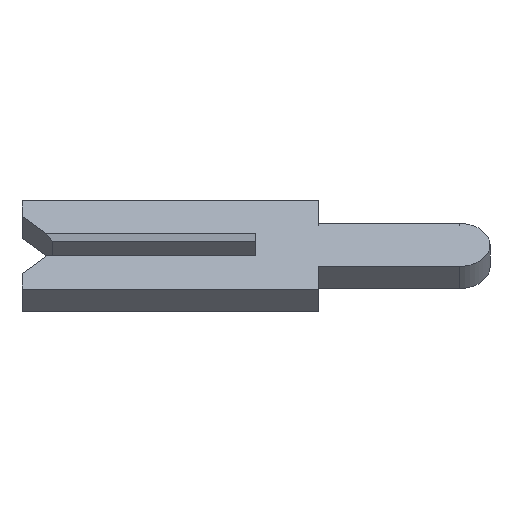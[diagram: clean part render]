
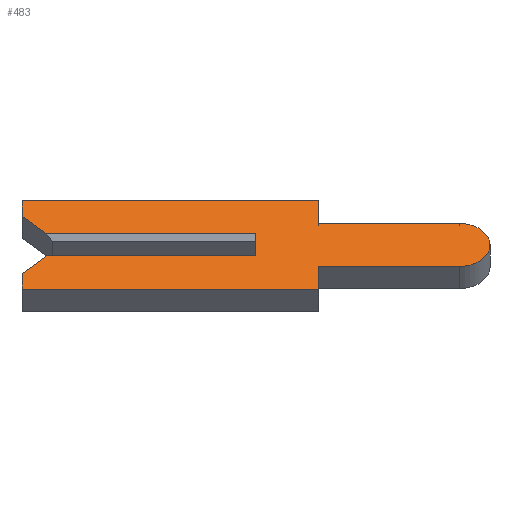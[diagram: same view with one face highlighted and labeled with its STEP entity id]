
A CAD part, left-side view. The second image highlights one B-rep face of the part: STEP entity #483.
In plain terms, the highlighted face is planar.
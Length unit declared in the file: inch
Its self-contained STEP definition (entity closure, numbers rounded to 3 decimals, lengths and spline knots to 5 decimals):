
#17 = LINE ( 'NONE', #976, #556 ) ;
#19 = DIRECTION ( 'NONE',  ( 0., 0., 1. ) ) ;
#25 = VECTOR ( 'NONE', #899, 39.37008 ) ;
#27 = CARTESIAN_POINT ( 'NONE',  ( -0.01, 0.1305, -0.0065 ) ) ;
#33 = VERTEX_POINT ( 'NONE', #515 ) ;
#41 = LINE ( 'NONE', #292, #130 ) ;
#45 = VECTOR ( 'NONE', #214, 39.37008 ) ;
#46 = EDGE_LOOP ( 'NONE', ( #150, #789, #1034, #420, #345, #579, #1049, #312, #749, #399, #894, #68, #518, #466 ) ) ;
#61 = AXIS2_PLACEMENT_3D ( 'NONE', #661, #928, #525 ) ;
#62 = EDGE_CURVE ( 'NONE', #847, #322, #457, .T. ) ;
#68 = ORIENTED_EDGE ( 'NONE', *, *, #182, .F. ) ;
#73 = CARTESIAN_POINT ( 'NONE',  ( -0.01, -0.04, 0.0195 ) ) ;
#76 = CARTESIAN_POINT ( 'NONE',  ( -0.01, -0.04, -0.0195 ) ) ;
#97 = EDGE_CURVE ( 'NONE', #671, #924, #884, .T. ) ;
#107 = CARTESIAN_POINT ( 'NONE',  ( -0.01, -0.04, 0.0195 ) ) ;
#108 = VERTEX_POINT ( 'NONE', #359 ) ;
#111 = DIRECTION ( 'NONE',  ( 0., -0.707, 0.707 ) ) ;
#122 = CARTESIAN_POINT ( 'NONE',  ( -0.01, -0.1305, 0.0195 ) ) ;
#126 = FACE_OUTER_BOUND ( 'NONE', #46, .T. ) ;
#130 = VECTOR ( 'NONE', #450, 39.37008 ) ;
#150 = ORIENTED_EDGE ( 'NONE', *, *, #632, .T. ) ;
#168 = DIRECTION ( 'NONE',  ( 0., 0., -1. ) ) ;
#177 = CARTESIAN_POINT ( 'NONE',  ( -0.01, -0.04, -0.0195 ) ) ;
#182 = EDGE_CURVE ( 'NONE', #686, #671, #241, .T. ) ;
#196 = EDGE_CURVE ( 'NONE', #33, #621, #849, .T. ) ;
#202 = VECTOR ( 'NONE', #812, 39.37008 ) ;
#214 = DIRECTION ( 'NONE',  ( 0., -1., 0. ) ) ;
#241 = LINE ( 'NONE', #433, #998 ) ;
#254 = VECTOR ( 'NONE', #352, 39.37008 ) ;
#264 = DIRECTION ( 'NONE',  ( 0., 1., 0. ) ) ;
#290 = CARTESIAN_POINT ( 'NONE',  ( -0.01, 0.15, -0.04 ) ) ;
#291 = CARTESIAN_POINT ( 'NONE',  ( -0.01, 0., 0.0065 ) ) ;
#292 = CARTESIAN_POINT ( 'NONE',  ( -0.01, 0.15, 0.026 ) ) ;
#309 = EDGE_CURVE ( 'NONE', #108, #686, #41, .T. ) ;
#312 = ORIENTED_EDGE ( 'NONE', *, *, #571, .F. ) ;
#322 = VERTEX_POINT ( 'NONE', #872 ) ;
#328 = CARTESIAN_POINT ( 'NONE',  ( -0.01, 0.134, 0.01 ) ) ;
#345 = ORIENTED_EDGE ( 'NONE', *, *, #1066, .F. ) ;
#352 = DIRECTION ( 'NONE',  ( 0., 1., 0. ) ) ;
#359 = CARTESIAN_POINT ( 'NONE',  ( -0.01, 0.15, 0.026 ) ) ;
#363 = CARTESIAN_POINT ( 'NONE',  ( -0.01, -0.1305, -0.0195 ) ) ;
#395 = PLANE ( 'NONE',  #596 ) ;
#399 = ORIENTED_EDGE ( 'NONE', *, *, #594, .F. ) ;
#420 = ORIENTED_EDGE ( 'NONE', *, *, #1006, .F. ) ;
#421 = VERTEX_POINT ( 'NONE', #122 ) ;
#430 = VECTOR ( 'NONE', #1085, 39.37008 ) ;
#433 = CARTESIAN_POINT ( 'NONE',  ( -0.01, 0.15, 0.04 ) ) ;
#434 = EDGE_CURVE ( 'NONE', #479, #108, #929, .T. ) ;
#450 = DIRECTION ( 'NONE',  ( 0., 0., 1. ) ) ;
#457 = LINE ( 'NONE', #1031, #767 ) ;
#460 = CARTESIAN_POINT ( 'NONE',  ( -0.01, -0.1305, -0.01 ) ) ;
#466 = ORIENTED_EDGE ( 'NONE', *, *, #434, .F. ) ;
#479 = VERTEX_POINT ( 'NONE', #328 ) ;
#483 = ADVANCED_FACE ( 'NONE', ( #126 ), #395, .F. ) ;
#485 = DIRECTION ( 'NONE',  ( 1., 0., 0. ) ) ;
#505 = VECTOR ( 'NONE', #111, 39.37008 ) ;
#514 = VECTOR ( 'NONE', #264, 39.37008 ) ;
#515 = CARTESIAN_POINT ( 'NONE',  ( -0.01, 0., -0.01 ) ) ;
#518 = ORIENTED_EDGE ( 'NONE', *, *, #309, .F. ) ;
#519 = VERTEX_POINT ( 'NONE', #915 ) ;
#522 = VECTOR ( 'NONE', #19, 39.37008 ) ;
#525 = DIRECTION ( 'NONE',  ( 0., 0., -1. ) ) ;
#553 = CARTESIAN_POINT ( 'NONE',  ( -0.01, 0.1305, 0.0065 ) ) ;
#556 = VECTOR ( 'NONE', #869, 39.37008 ) ;
#568 = CARTESIAN_POINT ( 'NONE',  ( -0.01, 0., 0.01 ) ) ;
#571 = EDGE_CURVE ( 'NONE', #941, #847, #645, .T. ) ;
#579 = ORIENTED_EDGE ( 'NONE', *, *, #1028, .F. ) ;
#594 = EDGE_CURVE ( 'NONE', #924, #421, #746, .T. ) ;
#595 = DIRECTION ( 'NONE',  ( 0., 0., -1. ) ) ;
#596 = AXIS2_PLACEMENT_3D ( 'NONE', #985, #485, #168 ) ;
#621 = VERTEX_POINT ( 'NONE', #568 ) ;
#632 = EDGE_CURVE ( 'NONE', #479, #621, #799, .T. ) ;
#645 = LINE ( 'NONE', #76, #514 ) ;
#647 = VECTOR ( 'NONE', #595, 39.37008 ) ;
#661 = CARTESIAN_POINT ( 'NONE',  ( -0.01, -0.1305, 0. ) ) ;
#671 = VERTEX_POINT ( 'NONE', #729 ) ;
#675 = CARTESIAN_POINT ( 'NONE',  ( -0.01, 0.134, -0.01 ) ) ;
#686 = VERTEX_POINT ( 'NONE', #922 ) ;
#729 = CARTESIAN_POINT ( 'NONE',  ( -0.01, -0.04, 0.04 ) ) ;
#746 = LINE ( 'NONE', #73, #202 ) ;
#749 = ORIENTED_EDGE ( 'NONE', *, *, #840, .F. ) ;
#756 = CARTESIAN_POINT ( 'NONE',  ( -0.01, -0.04, 0.04 ) ) ;
#762 = CARTESIAN_POINT ( 'NONE',  ( -0.01, 0.15, -0.026 ) ) ;
#767 = VECTOR ( 'NONE', #1042, 39.37008 ) ;
#778 = CIRCLE ( 'NONE', #61, 0.0195 ) ;
#789 = ORIENTED_EDGE ( 'NONE', *, *, #196, .F. ) ;
#799 = LINE ( 'NONE', #908, #430 ) ;
#812 = DIRECTION ( 'NONE',  ( 0., -1., 0. ) ) ;
#840 = EDGE_CURVE ( 'NONE', #421, #941, #778, .T. ) ;
#847 = VERTEX_POINT ( 'NONE', #177 ) ;
#849 = LINE ( 'NONE', #291, #522 ) ;
#862 = VERTEX_POINT ( 'NONE', #762 ) ;
#869 = DIRECTION ( 'NONE',  ( 0., 0., 1. ) ) ;
#872 = CARTESIAN_POINT ( 'NONE',  ( -0.01, -0.04, -0.04 ) ) ;
#884 = LINE ( 'NONE', #756, #647 ) ;
#894 = ORIENTED_EDGE ( 'NONE', *, *, #97, .F. ) ;
#899 = DIRECTION ( 'NONE',  ( 0., 0.707, 0.707 ) ) ;
#908 = CARTESIAN_POINT ( 'NONE',  ( -0.01, 0.15, 0.01 ) ) ;
#915 = CARTESIAN_POINT ( 'NONE',  ( -0.01, 0.15, -0.04 ) ) ;
#922 = CARTESIAN_POINT ( 'NONE',  ( -0.01, 0.15, 0.04 ) ) ;
#924 = VERTEX_POINT ( 'NONE', #107 ) ;
#925 = VERTEX_POINT ( 'NONE', #675 ) ;
#928 = DIRECTION ( 'NONE',  ( 1., 0., 0. ) ) ;
#929 = LINE ( 'NONE', #553, #25 ) ;
#940 = DIRECTION ( 'NONE',  ( 0., -1., 0. ) ) ;
#941 = VERTEX_POINT ( 'NONE', #363 ) ;
#967 = LINE ( 'NONE', #27, #505 ) ;
#976 = CARTESIAN_POINT ( 'NONE',  ( -0.01, 0.15, -0.026 ) ) ;
#985 = CARTESIAN_POINT ( 'NONE',  ( -0.01, -0.1305, 0. ) ) ;
#998 = VECTOR ( 'NONE', #940, 39.37008 ) ;
#1006 = EDGE_CURVE ( 'NONE', #862, #925, #967, .T. ) ;
#1015 = LINE ( 'NONE', #460, #45 ) ;
#1028 = EDGE_CURVE ( 'NONE', #322, #519, #1052, .T. ) ;
#1031 = CARTESIAN_POINT ( 'NONE',  ( -0.01, -0.04, -0.04 ) ) ;
#1034 = ORIENTED_EDGE ( 'NONE', *, *, #1080, .F. ) ;
#1042 = DIRECTION ( 'NONE',  ( 0., 0., -1. ) ) ;
#1049 = ORIENTED_EDGE ( 'NONE', *, *, #62, .F. ) ;
#1052 = LINE ( 'NONE', #290, #254 ) ;
#1066 = EDGE_CURVE ( 'NONE', #519, #862, #17, .T. ) ;
#1080 = EDGE_CURVE ( 'NONE', #925, #33, #1015, .T. ) ;
#1085 = DIRECTION ( 'NONE',  ( 0., -1., 0. ) ) ;
